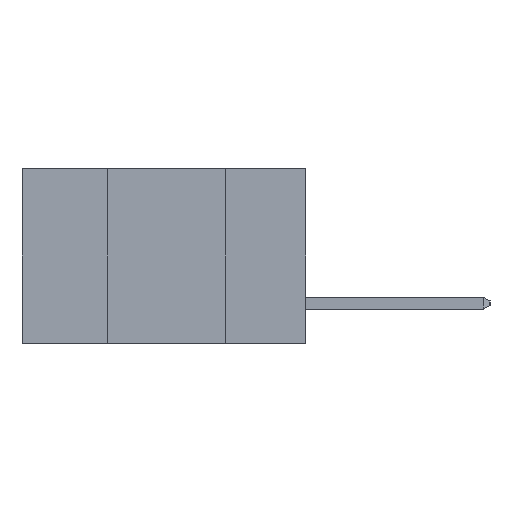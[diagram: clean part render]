
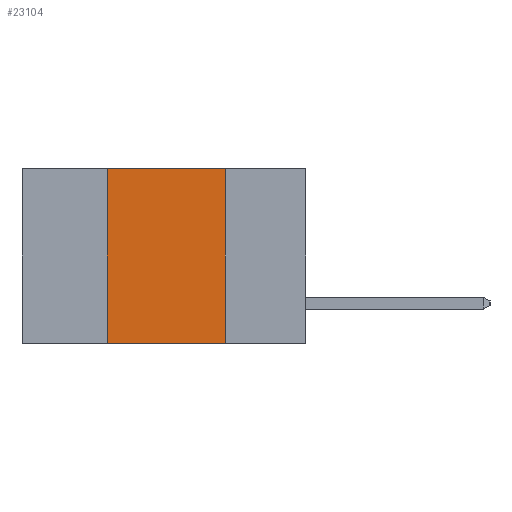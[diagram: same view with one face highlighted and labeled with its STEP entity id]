
A CAD part, left-side view. The second image highlights one B-rep face of the part: STEP entity #23104.
In plain terms, the highlighted planar face has unit normal (-1, 0, 0).
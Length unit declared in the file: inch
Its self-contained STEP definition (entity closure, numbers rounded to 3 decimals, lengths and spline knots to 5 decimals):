
#718 = VERTEX_POINT ( 'NONE', #4153 ) ;
#973 = VERTEX_POINT ( 'NONE', #6822 ) ;
#1384 = CARTESIAN_POINT ( 'NONE',  ( 0., 0.6, 0. ) ) ;
#1589 = ORIENTED_EDGE ( 'NONE', *, *, #4509, .F. ) ;
#2213 = EDGE_CURVE ( 'NONE', #973, #22883, #25701, .T. ) ;
#2497 = VERTEX_POINT ( 'NONE', #22252 ) ;
#2541 = FACE_OUTER_BOUND ( 'NONE', #22201, .T. ) ;
#4153 = CARTESIAN_POINT ( 'NONE',  ( 0., 0.17, -0.37 ) ) ;
#4509 = EDGE_CURVE ( 'NONE', #2497, #973, #4795, .T. ) ;
#4795 = LINE ( 'NONE', #21567, #17780 ) ;
#5116 = EDGE_CURVE ( 'NONE', #2497, #718, #18870, .T. ) ;
#6822 = CARTESIAN_POINT ( 'NONE',  ( 0., 0.42, 0. ) ) ;
#11064 = ORIENTED_EDGE ( 'NONE', *, *, #5116, .T. ) ;
#11684 = PLANE ( 'NONE',  #15809 ) ;
#13434 = CARTESIAN_POINT ( 'NONE',  ( 0., 0.17, 0. ) ) ;
#14158 = DIRECTION ( 'NONE',  ( 0., 0., -1. ) ) ;
#15809 = AXIS2_PLACEMENT_3D ( 'NONE', #18934, #28575, #14158 ) ;
#16738 = ORIENTED_EDGE ( 'NONE', *, *, #18436, .F. ) ;
#16862 = VECTOR ( 'NONE', #24509, 39.37008 ) ;
#16870 = CARTESIAN_POINT ( 'NONE',  ( 0., 0.6, -0.37 ) ) ;
#16892 = DIRECTION ( 'NONE',  ( 0., -1., 0. ) ) ;
#17613 = DIRECTION ( 'NONE',  ( 0., -1., 0. ) ) ;
#17780 = VECTOR ( 'NONE', #21414, 39.37008 ) ;
#18436 = EDGE_CURVE ( 'NONE', #22883, #718, #23281, .T. ) ;
#18870 = LINE ( 'NONE', #16870, #24532 ) ;
#18934 = CARTESIAN_POINT ( 'NONE',  ( 0., 0.6, 0. ) ) ;
#19856 = ORIENTED_EDGE ( 'NONE', *, *, #2213, .F. ) ;
#21414 = DIRECTION ( 'NONE',  ( 0., 0., 1. ) ) ;
#21567 = CARTESIAN_POINT ( 'NONE',  ( 0., 0.42, 0. ) ) ;
#22201 = EDGE_LOOP ( 'NONE', ( #16738, #19856, #1589, #11064 ) ) ;
#22252 = CARTESIAN_POINT ( 'NONE',  ( 0., 0.42, -0.37 ) ) ;
#22883 = VERTEX_POINT ( 'NONE', #13434 ) ;
#23104 = ADVANCED_FACE ( 'NONE', ( #2541 ), #11684, .F. ) ;
#23281 = LINE ( 'NONE', #26815, #16862 ) ;
#24509 = DIRECTION ( 'NONE',  ( 0., 0., -1. ) ) ;
#24532 = VECTOR ( 'NONE', #16892, 39.37008 ) ;
#25701 = LINE ( 'NONE', #1384, #31259 ) ;
#26815 = CARTESIAN_POINT ( 'NONE',  ( 0., 0.17, 0. ) ) ;
#28575 = DIRECTION ( 'NONE',  ( 1., 0., 0. ) ) ;
#31259 = VECTOR ( 'NONE', #17613, 39.37008 ) ;
